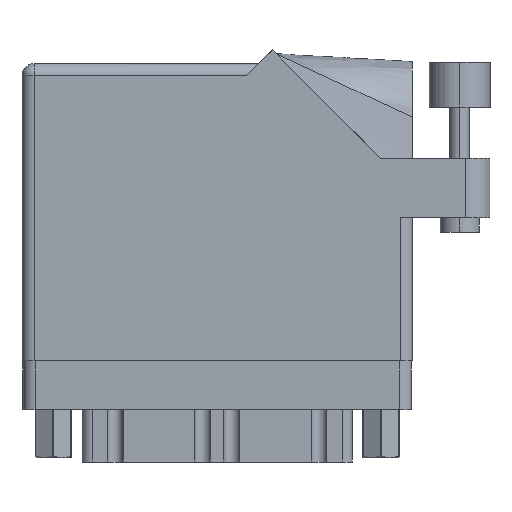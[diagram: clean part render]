
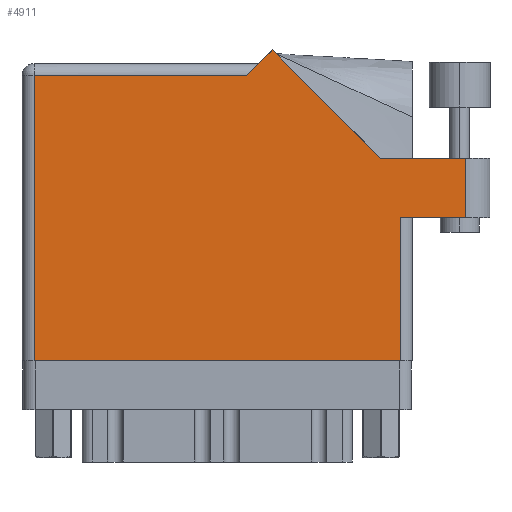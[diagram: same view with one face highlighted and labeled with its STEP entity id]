
A CAD part, front view. The second image highlights one B-rep face of the part: STEP entity #4911.
In plain terms, the highlighted face is planar.
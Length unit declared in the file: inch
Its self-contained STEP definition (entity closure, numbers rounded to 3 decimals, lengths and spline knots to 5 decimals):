
#81 = DIRECTION ( 'NONE',  ( -1., 0., 0. ) ) ;
#1074 = CARTESIAN_POINT ( 'NONE',  ( 2.41, 1.044, 0. ) ) ;
#1303 = DIRECTION ( 'NONE',  ( -1., 0., 0. ) ) ;
#2006 = VERTEX_POINT ( 'NONE', #13286 ) ;
#2693 = VECTOR ( 'NONE', #9204, 39.37008 ) ;
#2980 = DIRECTION ( 'NONE',  ( 1., 0., 0. ) ) ;
#3299 = CARTESIAN_POINT ( 'NONE',  ( 2.285, 1.044, 0. ) ) ;
#3856 = LINE ( 'NONE', #11272, #38489 ) ;
#4158 = CARTESIAN_POINT ( 'NONE',  ( 0., 1.468, 0. ) ) ;
#4911 = ADVANCED_FACE ( 'NONE', ( #30808 ), #45460, .F. ) ;
#5078 = CARTESIAN_POINT ( 'NONE',  ( 1.948, 0.737, 0. ) ) ;
#5160 = CARTESIAN_POINT ( 'NONE',  ( 1.948, 0.737, 0. ) ) ;
#5281 = DIRECTION ( 'NONE',  ( 1., 0., 0. ) ) ;
#6063 = ORIENTED_EDGE ( 'NONE', *, *, #39446, .T. ) ;
#7210 = ORIENTED_EDGE ( 'NONE', *, *, #45316, .T. ) ;
#7972 = ORIENTED_EDGE ( 'NONE', *, *, #23952, .T. ) ;
#8350 = VECTOR ( 'NONE', #28201, 39.37008 ) ;
#8955 = DIRECTION ( 'NONE',  ( 0., 0., -1. ) ) ;
#8970 = LINE ( 'NONE', #5160, #2693 ) ;
#9204 = DIRECTION ( 'NONE',  ( 0., 1., 0. ) ) ;
#9654 = VERTEX_POINT ( 'NONE', #32525 ) ;
#9743 = EDGE_CURVE ( 'NONE', #14980, #39105, #30326, .T. ) ;
#11272 = CARTESIAN_POINT ( 'NONE',  ( 1.84442, 1.044, 0. ) ) ;
#12186 = CARTESIAN_POINT ( 'NONE',  ( 1.217, 1.53, 0. ) ) ;
#12583 = ORIENTED_EDGE ( 'NONE', *, *, #41903, .T. ) ;
#13163 = VERTEX_POINT ( 'NONE', #13595 ) ;
#13286 = CARTESIAN_POINT ( 'NONE',  ( 1.28771, 1.60071, 0. ) ) ;
#13339 = LINE ( 'NONE', #23910, #8350 ) ;
#13595 = CARTESIAN_POINT ( 'NONE',  ( 2.285, 0.737, 0. ) ) ;
#14241 = CARTESIAN_POINT ( 'NONE',  ( 0., 0., 0. ) ) ;
#14980 = VERTEX_POINT ( 'NONE', #3299 ) ;
#15897 = EDGE_LOOP ( 'NONE', ( #7210, #24432, #35951, #25927, #29404, #6063, #7972, #29627, #12583 ) ) ;
#16753 = VERTEX_POINT ( 'NONE', #33555 ) ;
#17378 = LINE ( 'NONE', #14241, #29554 ) ;
#18069 = LINE ( 'NONE', #4158, #29349 ) ;
#21604 = LINE ( 'NONE', #39133, #24005 ) ;
#23910 = CARTESIAN_POINT ( 'NONE',  ( 0.062, 0., 0. ) ) ;
#23952 = EDGE_CURVE ( 'NONE', #36663, #34211, #13339, .T. ) ;
#24005 = VECTOR ( 'NONE', #31921, 39.37008 ) ;
#24158 = VECTOR ( 'NONE', #37404, 39.37008 ) ;
#24432 = ORIENTED_EDGE ( 'NONE', *, *, #30526, .T. ) ;
#25927 = ORIENTED_EDGE ( 'NONE', *, *, #35950, .T. ) ;
#26742 = CARTESIAN_POINT ( 'NONE',  ( 1.84442, 1.044, 0. ) ) ;
#28201 = DIRECTION ( 'NONE',  ( 0., -1., 0. ) ) ;
#28885 = CARTESIAN_POINT ( 'NONE',  ( 0.062, 0., 0. ) ) ;
#29349 = VECTOR ( 'NONE', #81, 39.37008 ) ;
#29404 = ORIENTED_EDGE ( 'NONE', *, *, #41683, .T. ) ;
#29554 = VECTOR ( 'NONE', #2980, 39.37008 ) ;
#29627 = ORIENTED_EDGE ( 'NONE', *, *, #42961, .T. ) ;
#29797 = VECTOR ( 'NONE', #5281, 39.37008 ) ;
#30326 = LINE ( 'NONE', #1074, #36844 ) ;
#30526 = EDGE_CURVE ( 'NONE', #13163, #14980, #21604, .T. ) ;
#30808 = FACE_OUTER_BOUND ( 'NONE', #15897, .T. ) ;
#31045 = DIRECTION ( 'NONE',  ( -1., 0., 0. ) ) ;
#31921 = DIRECTION ( 'NONE',  ( 0., 1., 0. ) ) ;
#32525 = CARTESIAN_POINT ( 'NONE',  ( 1.948, 0., 0. ) ) ;
#33555 = CARTESIAN_POINT ( 'NONE',  ( 1.155, 1.468, 0. ) ) ;
#34211 = VERTEX_POINT ( 'NONE', #28885 ) ;
#34439 = VERTEX_POINT ( 'NONE', #5078 ) ;
#35263 = CARTESIAN_POINT ( 'NONE',  ( 2.01, 0.737, 0. ) ) ;
#35950 = EDGE_CURVE ( 'NONE', #39105, #2006, #3856, .T. ) ;
#35951 = ORIENTED_EDGE ( 'NONE', *, *, #9743, .T. ) ;
#36663 = VERTEX_POINT ( 'NONE', #46490 ) ;
#36844 = VECTOR ( 'NONE', #1303, 39.37008 ) ;
#37404 = DIRECTION ( 'NONE',  ( -0.707, -0.707, 0. ) ) ;
#37696 = LINE ( 'NONE', #35263, #29797 ) ;
#38489 = VECTOR ( 'NONE', #44165, 39.37008 ) ;
#39105 = VERTEX_POINT ( 'NONE', #26742 ) ;
#39133 = CARTESIAN_POINT ( 'NONE',  ( 2.285, 1.044, 0. ) ) ;
#39446 = EDGE_CURVE ( 'NONE', #16753, #36663, #18069, .T. ) ;
#40329 = AXIS2_PLACEMENT_3D ( 'NONE', #41851, #8955, #31045 ) ;
#41683 = EDGE_CURVE ( 'NONE', #2006, #16753, #45324, .T. ) ;
#41851 = CARTESIAN_POINT ( 'NONE',  ( 0., 1.53, 0. ) ) ;
#41903 = EDGE_CURVE ( 'NONE', #9654, #34439, #8970, .T. ) ;
#42961 = EDGE_CURVE ( 'NONE', #34211, #9654, #17378, .T. ) ;
#44165 = DIRECTION ( 'NONE',  ( -0.707, 0.707, 0. ) ) ;
#45316 = EDGE_CURVE ( 'NONE', #34439, #13163, #37696, .T. ) ;
#45324 = LINE ( 'NONE', #12186, #24158 ) ;
#45460 = PLANE ( 'NONE',  #40329 ) ;
#46490 = CARTESIAN_POINT ( 'NONE',  ( 0.062, 1.468, 0. ) ) ;
